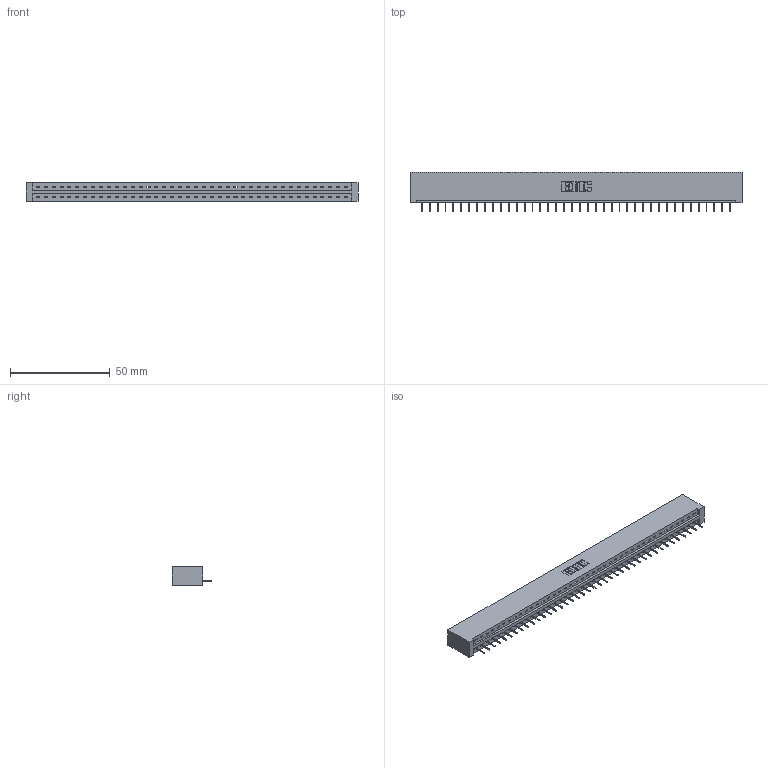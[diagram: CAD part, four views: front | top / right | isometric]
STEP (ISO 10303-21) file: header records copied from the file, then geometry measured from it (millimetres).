
FILE_DESCRIPTION (( 'STEP AP203' ), '1' );
FILE_NAME ('387-040-524-101.STEP', '2018-09-19T10:26:23', ( '' ), ( '' ), 'SwSTEP 2.0', 'SolidWorks 2016', '' );
FILE_SCHEMA (( 'CONFIG_CONTROL_DESIGN' ));
Length unit declared in the file: inch
Products named in the file (3): 387-040-524-101; 337 Part_No Mounting Lugs; 345-292-001_345-293-124
Assembly tree (41 placements, depth 2):
  387-040-524-101
    337 Part_No Mounting Lugs
    345-292-001_345-293-124  x40
Bounding box: 166.37 x 19.69 x 9.4 mm (x, y, z)
Volume: 17847 mm3; surface area: 17856.9 mm2
Topology: 41 solids, 41 shells, 2746 faces, 7967 edges, 5150 vertices
Faces by surface type: plane 2146, cylinder 600
Entity records: 29789 total; most frequent: CARTESIAN_POINT 5194, ORIENTED_EDGE 5170, DIRECTION 4369, EDGE_CURVE 2585, LINE 2469, VECTOR 2469, VERTEX_POINT 1718, AXIS2_PLACEMENT_3D 950
